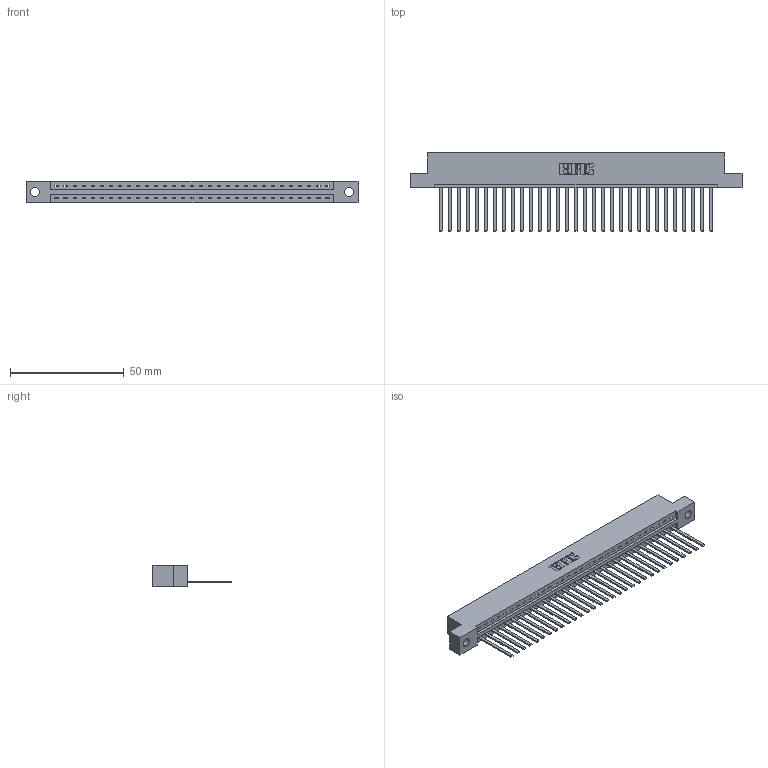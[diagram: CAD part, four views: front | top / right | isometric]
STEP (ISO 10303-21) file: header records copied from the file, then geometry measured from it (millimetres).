
FILE_DESCRIPTION (( 'STEP AP203' ), '1' );
FILE_NAME ('387-031-544-104.STEP', '2019-10-03T19:45:36', ( '' ), ( '' ), 'SwSTEP 2.0', 'SolidWorks 2016', '' );
FILE_SCHEMA (( 'CONFIG_CONTROL_DESIGN' ));
Length unit declared in the file: inch
Products named in the file (3): 345-292-001_345-293-144; 337 Part_Flush Mounting Lugs - 0.156 Dia-TH; 387-031-544-104
Assembly tree (32 placements, depth 2):
  387-031-544-104
    337 Part_Flush Mounting Lugs - 0.156 Dia-TH
    345-292-001_345-293-144  x31
Bounding box: 145.85 x 34.3 x 9.4 mm (x, y, z)
Volume: 15291.8 mm3; surface area: 16717.1 mm2
Topology: 32 solids, 32 shells, 1850 faces, 5581 edges, 3678 vertices
Faces by surface type: plane 1372, cylinder 478
Entity records: 24285 total; most frequent: CARTESIAN_POINT 4235, ORIENTED_EDGE 4202, DIRECTION 3583, EDGE_CURVE 2101, LINE 1977, VECTOR 1977, VERTEX_POINT 1398, AXIS2_PLACEMENT_3D 803
